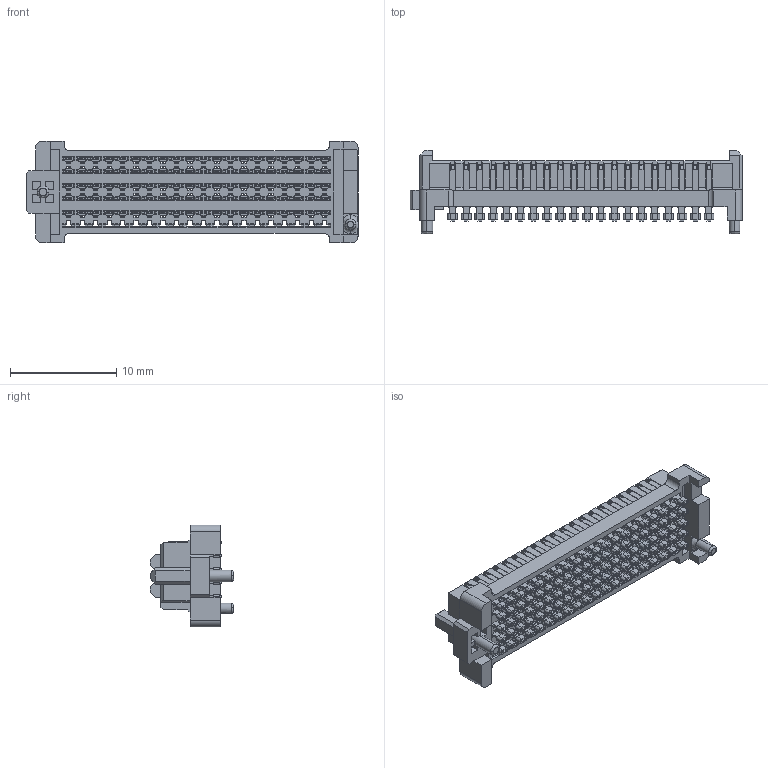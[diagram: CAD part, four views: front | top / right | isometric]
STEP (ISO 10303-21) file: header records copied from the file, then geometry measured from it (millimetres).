
FILE_DESCRIPTION (( 'STEP AP214' ), '1' );
FILE_NAME ('470-100-529-001.STEP', '2020-05-19T17:09:11', ( '' ), ( '' ), 'SwSTEP 2.0', 'SolidWorks 2020', '' );
FILE_SCHEMA (( 'AUTOMOTIVE_DESIGN' ));
Length unit declared in the file: millimetre
Products named in the file (4): 470-100-529-001; 470-100-529-001 CON; 470-100-529-001 COL; 470-100-529-001 INS
Assembly tree (201 placements, depth 2):
  470-100-529-001
    470-100-529-001 INS
    470-100-529-001 CON  x100
    470-100-529-001 COL  x100
Bounding box: 31.28 x 7.88 x 9.6 mm (x, y, z)
Volume: 671 mm3; surface area: 3198.4 mm2
Topology: 201 solids, 201 shells, 10598 faces, 29197 edges, 18887 vertices
Faces by surface type: plane 7897, cylinder 2695, bspline 6
Entity records: 96772 total; most frequent: CARTESIAN_POINT 17609, ORIENTED_EDGE 17012, DIRECTION 14881, EDGE_CURVE 8506, LINE 8231, VECTOR 8231, VERTEX_POINT 5423, AXIS2_PLACEMENT_3D 3325
